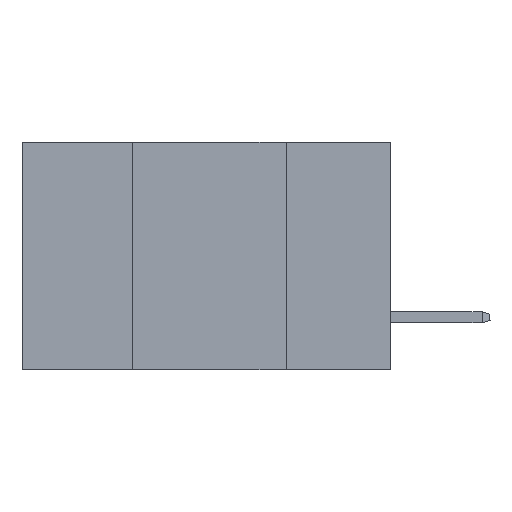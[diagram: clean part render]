
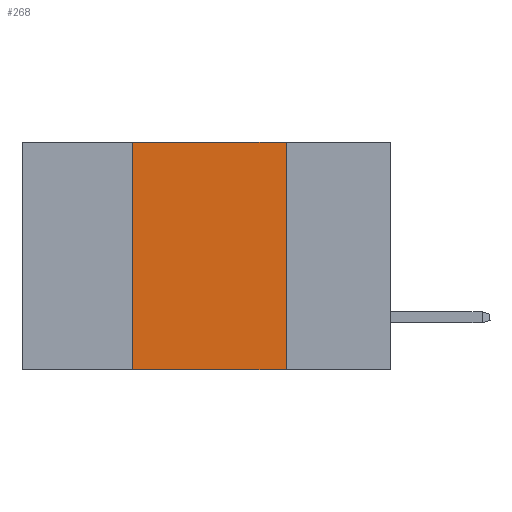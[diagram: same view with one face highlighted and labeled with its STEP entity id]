
A CAD part, left-side view. The second image highlights one B-rep face of the part: STEP entity #268.
In plain terms, the highlighted planar face has unit normal (-1, 0, 0).
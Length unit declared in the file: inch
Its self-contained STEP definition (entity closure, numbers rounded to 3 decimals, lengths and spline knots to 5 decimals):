
#135 = VECTOR ( 'NONE', #5113, 39.37008 ) ;
#268 = ADVANCED_FACE ( 'NONE', ( #37192 ), #8874, .F. ) ;
#1492 = CARTESIAN_POINT ( 'NONE',  ( 0., 0.17, 0. ) ) ;
#4451 = EDGE_CURVE ( 'NONE', #7706, #7791, #40132, .T. ) ;
#4737 = CARTESIAN_POINT ( 'NONE',  ( 0., 0.6, -0.37 ) ) ;
#5113 = DIRECTION ( 'NONE',  ( 0., 0., -1. ) ) ;
#5346 = AXIS2_PLACEMENT_3D ( 'NONE', #18244, #5675, #11761 ) ;
#5455 = EDGE_CURVE ( 'NONE', #18801, #26322, #37661, .T. ) ;
#5675 = DIRECTION ( 'NONE',  ( 1., 0., 0. ) ) ;
#7232 = CARTESIAN_POINT ( 'NONE',  ( 0., 0.17, 0. ) ) ;
#7706 = VERTEX_POINT ( 'NONE', #26413 ) ;
#7791 = VERTEX_POINT ( 'NONE', #7232 ) ;
#8874 = PLANE ( 'NONE',  #5346 ) ;
#9851 = EDGE_LOOP ( 'NONE', ( #27949, #32281, #22164, #36977 ) ) ;
#10788 = EDGE_CURVE ( 'NONE', #7791, #26322, #26891, .T. ) ;
#11761 = DIRECTION ( 'NONE',  ( 0., 0., -1. ) ) ;
#14426 = DIRECTION ( 'NONE',  ( 0., -1., 0. ) ) ;
#18244 = CARTESIAN_POINT ( 'NONE',  ( 0., 0.6, 0. ) ) ;
#18801 = VERTEX_POINT ( 'NONE', #35965 ) ;
#21445 = VECTOR ( 'NONE', #33818, 39.37008 ) ;
#22164 = ORIENTED_EDGE ( 'NONE', *, *, #38613, .F. ) ;
#26322 = VERTEX_POINT ( 'NONE', #38503 ) ;
#26363 = LINE ( 'NONE', #33258, #21445 ) ;
#26413 = CARTESIAN_POINT ( 'NONE',  ( 0., 0.42, 0. ) ) ;
#26891 = LINE ( 'NONE', #1492, #135 ) ;
#27548 = DIRECTION ( 'NONE',  ( 0., -1., 0. ) ) ;
#27949 = ORIENTED_EDGE ( 'NONE', *, *, #10788, .F. ) ;
#31740 = VECTOR ( 'NONE', #27548, 39.37008 ) ;
#32281 = ORIENTED_EDGE ( 'NONE', *, *, #4451, .F. ) ;
#32675 = VECTOR ( 'NONE', #14426, 39.37008 ) ;
#33258 = CARTESIAN_POINT ( 'NONE',  ( 0., 0.42, 0. ) ) ;
#33818 = DIRECTION ( 'NONE',  ( 0., 0., 1. ) ) ;
#35965 = CARTESIAN_POINT ( 'NONE',  ( 0., 0.42, -0.37 ) ) ;
#36977 = ORIENTED_EDGE ( 'NONE', *, *, #5455, .T. ) ;
#37192 = FACE_OUTER_BOUND ( 'NONE', #9851, .T. ) ;
#37661 = LINE ( 'NONE', #4737, #32675 ) ;
#38503 = CARTESIAN_POINT ( 'NONE',  ( 0., 0.17, -0.37 ) ) ;
#38613 = EDGE_CURVE ( 'NONE', #18801, #7706, #26363, .T. ) ;
#39807 = CARTESIAN_POINT ( 'NONE',  ( 0., 0.6, 0. ) ) ;
#40132 = LINE ( 'NONE', #39807, #31740 ) ;
